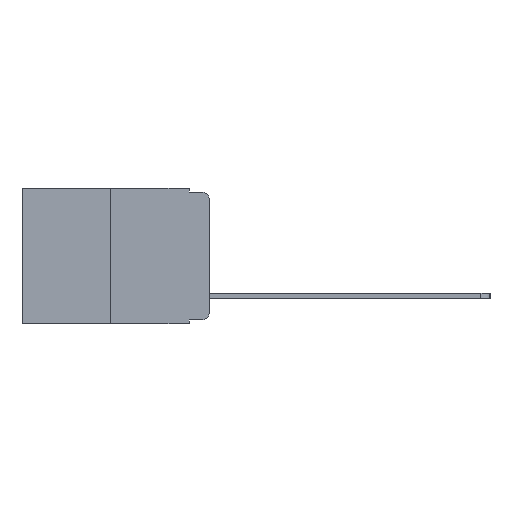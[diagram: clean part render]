
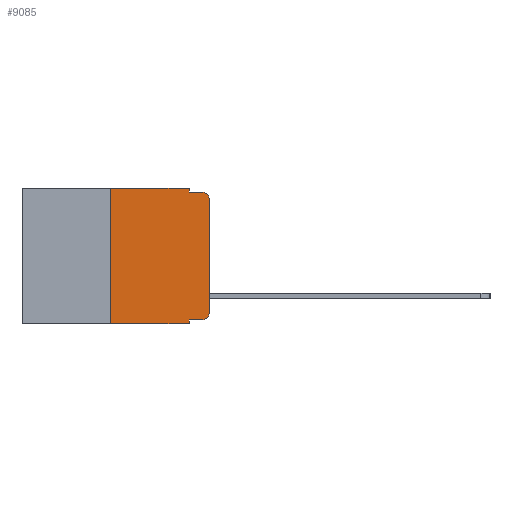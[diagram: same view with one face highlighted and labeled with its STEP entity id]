
A CAD part, left-side view. The second image highlights one B-rep face of the part: STEP entity #9085.
In plain terms, the highlighted planar face has unit normal (-1, 0, 0).
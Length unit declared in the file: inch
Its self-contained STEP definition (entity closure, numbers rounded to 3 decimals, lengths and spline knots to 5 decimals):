
#391 = VECTOR ( 'NONE', #4236, 39.37008 ) ;
#410 = CARTESIAN_POINT ( 'NONE',  ( 0., 0.051, -0.01 ) ) ;
#901 = DIRECTION ( 'NONE',  ( 0., 0., -1. ) ) ;
#932 = CARTESIAN_POINT ( 'NONE',  ( 0., 0.25, -0.343 ) ) ;
#972 = CARTESIAN_POINT ( 'NONE',  ( 0., 0., -0.03 ) ) ;
#1005 = CIRCLE ( 'NONE', #7547, 0.02 ) ;
#1157 = LINE ( 'NONE', #6272, #6333 ) ;
#1278 = LINE ( 'NONE', #9098, #10058 ) ;
#1353 = VECTOR ( 'NONE', #12919, 39.37008 ) ;
#1525 = LINE ( 'NONE', #3084, #391 ) ;
#1612 = DIRECTION ( 'NONE',  ( 0., -1., 0. ) ) ;
#1649 = DIRECTION ( 'NONE',  ( 0., -1., 0. ) ) ;
#1854 = VERTEX_POINT ( 'NONE', #9557 ) ;
#2108 = CARTESIAN_POINT ( 'NONE',  ( 0., 0.051, 0. ) ) ;
#2161 = VECTOR ( 'NONE', #3745, 39.37008 ) ;
#2199 = EDGE_CURVE ( 'NONE', #3920, #8246, #1278, .T. ) ;
#2622 = CARTESIAN_POINT ( 'NONE',  ( 0., 0.25, 0. ) ) ;
#2741 = CARTESIAN_POINT ( 'NONE',  ( 0., 0.02, -0.03 ) ) ;
#3084 = CARTESIAN_POINT ( 'NONE',  ( 0., 0., 0. ) ) ;
#3400 = ORIENTED_EDGE ( 'NONE', *, *, #11019, .F. ) ;
#3659 = VERTEX_POINT ( 'NONE', #972 ) ;
#3745 = DIRECTION ( 'NONE',  ( 0., 0., 1. ) ) ;
#3860 = DIRECTION ( 'NONE',  ( 0., 0., -1. ) ) ;
#3920 = VERTEX_POINT ( 'NONE', #7913 ) ;
#3927 = CARTESIAN_POINT ( 'NONE',  ( 0., 0.051, -0.333 ) ) ;
#4236 = DIRECTION ( 'NONE',  ( 0., 0., 1. ) ) ;
#4259 = CIRCLE ( 'NONE', #5517, 0.02 ) ;
#4261 = EDGE_CURVE ( 'NONE', #10527, #9319, #1005, .T. ) ;
#4439 = VERTEX_POINT ( 'NONE', #8722 ) ;
#4615 = VERTEX_POINT ( 'NONE', #932 ) ;
#4770 = CARTESIAN_POINT ( 'NONE',  ( 0., 0.051, 0. ) ) ;
#4814 = CARTESIAN_POINT ( 'NONE',  ( 0., 0.473, 0. ) ) ;
#4974 = EDGE_CURVE ( 'NONE', #1854, #10527, #7695, .T. ) ;
#5086 = LINE ( 'NONE', #9276, #10134 ) ;
#5517 = AXIS2_PLACEMENT_3D ( 'NONE', #2741, #9999, #3860 ) ;
#5799 = DIRECTION ( 'NONE',  ( 0., 0., -1. ) ) ;
#5842 = DIRECTION ( 'NONE',  ( 0., 0., -1. ) ) ;
#6005 = CARTESIAN_POINT ( 'NONE',  ( 0., 0.051, -0.01 ) ) ;
#6215 = VERTEX_POINT ( 'NONE', #410 ) ;
#6272 = CARTESIAN_POINT ( 'NONE',  ( 0., 0.051, 0. ) ) ;
#6333 = VECTOR ( 'NONE', #9345, 39.37008 ) ;
#6340 = EDGE_CURVE ( 'NONE', #1854, #4439, #1157, .T. ) ;
#6352 = EDGE_CURVE ( 'NONE', #9319, #3659, #1525, .T. ) ;
#6832 = LINE ( 'NONE', #6005, #1353 ) ;
#7500 = DIRECTION ( 'NONE',  ( -1., 0., 0. ) ) ;
#7536 = ORIENTED_EDGE ( 'NONE', *, *, #6352, .T. ) ;
#7542 = FACE_OUTER_BOUND ( 'NONE', #8493, .T. ) ;
#7547 = AXIS2_PLACEMENT_3D ( 'NONE', #13321, #7500, #901 ) ;
#7695 = LINE ( 'NONE', #3927, #12244 ) ;
#7867 = VECTOR ( 'NONE', #5799, 39.37008 ) ;
#7913 = CARTESIAN_POINT ( 'NONE',  ( 0., 0.25, 0. ) ) ;
#8246 = VERTEX_POINT ( 'NONE', #2108 ) ;
#8493 = EDGE_LOOP ( 'NONE', ( #7536, #11786, #3400, #11932, #12748, #8827, #11687, #11985, #10786, #11092 ) ) ;
#8722 = CARTESIAN_POINT ( 'NONE',  ( 0., 0.051, -0.343 ) ) ;
#8827 = ORIENTED_EDGE ( 'NONE', *, *, #9744, .F. ) ;
#9067 = EDGE_CURVE ( 'NONE', #8246, #6215, #13017, .T. ) ;
#9085 = ADVANCED_FACE ( 'NONE', ( #7542 ), #9839, .F. ) ;
#9098 = CARTESIAN_POINT ( 'NONE',  ( 0., 0.473, 0. ) ) ;
#9276 = CARTESIAN_POINT ( 'NONE',  ( 0., 0.473, -0.343 ) ) ;
#9319 = VERTEX_POINT ( 'NONE', #11152 ) ;
#9345 = DIRECTION ( 'NONE',  ( 0., 0., -1. ) ) ;
#9557 = CARTESIAN_POINT ( 'NONE',  ( 0., 0.051, -0.333 ) ) ;
#9744 = EDGE_CURVE ( 'NONE', #4615, #3920, #10455, .T. ) ;
#9839 = PLANE ( 'NONE',  #12069 ) ;
#9999 = DIRECTION ( 'NONE',  ( -1., 0., 0. ) ) ;
#10058 = VECTOR ( 'NONE', #1649, 39.37008 ) ;
#10134 = VECTOR ( 'NONE', #13102, 39.37008 ) ;
#10196 = CARTESIAN_POINT ( 'NONE',  ( 0., 0.02, -0.333 ) ) ;
#10291 = VERTEX_POINT ( 'NONE', #11711 ) ;
#10377 = EDGE_CURVE ( 'NONE', #3659, #10291, #4259, .T. ) ;
#10455 = LINE ( 'NONE', #2622, #2161 ) ;
#10527 = VERTEX_POINT ( 'NONE', #10196 ) ;
#10544 = EDGE_CURVE ( 'NONE', #4615, #4439, #5086, .T. ) ;
#10786 = ORIENTED_EDGE ( 'NONE', *, *, #4974, .T. ) ;
#11019 = EDGE_CURVE ( 'NONE', #6215, #10291, #6832, .T. ) ;
#11092 = ORIENTED_EDGE ( 'NONE', *, *, #4261, .T. ) ;
#11152 = CARTESIAN_POINT ( 'NONE',  ( 0., 0., -0.313 ) ) ;
#11687 = ORIENTED_EDGE ( 'NONE', *, *, #10544, .T. ) ;
#11711 = CARTESIAN_POINT ( 'NONE',  ( 0., 0.02, -0.01 ) ) ;
#11782 = DIRECTION ( 'NONE',  ( 1., 0., 0. ) ) ;
#11786 = ORIENTED_EDGE ( 'NONE', *, *, #10377, .T. ) ;
#11932 = ORIENTED_EDGE ( 'NONE', *, *, #9067, .F. ) ;
#11985 = ORIENTED_EDGE ( 'NONE', *, *, #6340, .F. ) ;
#12069 = AXIS2_PLACEMENT_3D ( 'NONE', #4814, #11782, #5842 ) ;
#12244 = VECTOR ( 'NONE', #1612, 39.37008 ) ;
#12748 = ORIENTED_EDGE ( 'NONE', *, *, #2199, .F. ) ;
#12919 = DIRECTION ( 'NONE',  ( 0., -1., 0. ) ) ;
#13017 = LINE ( 'NONE', #4770, #7867 ) ;
#13102 = DIRECTION ( 'NONE',  ( 0., -1., 0. ) ) ;
#13321 = CARTESIAN_POINT ( 'NONE',  ( 0., 0.02, -0.313 ) ) ;
